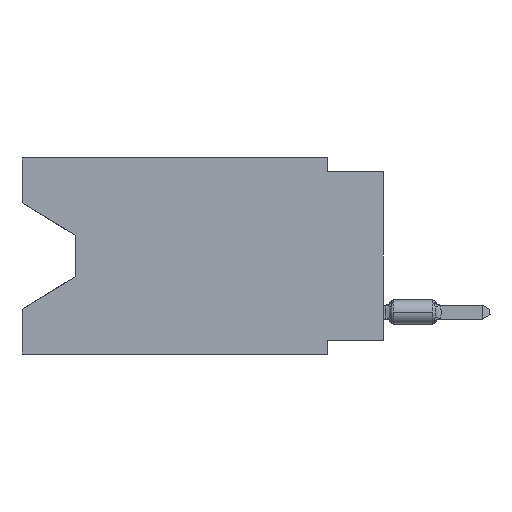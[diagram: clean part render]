
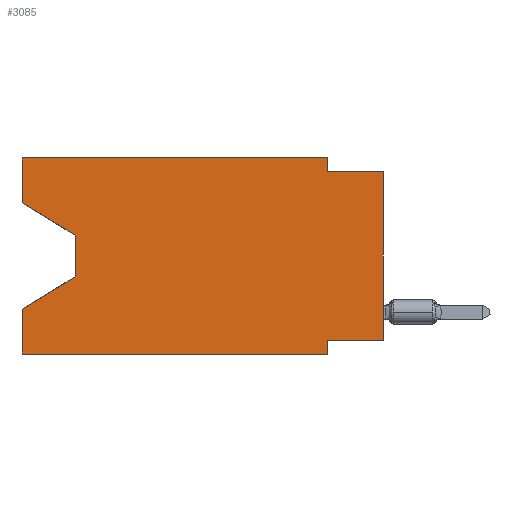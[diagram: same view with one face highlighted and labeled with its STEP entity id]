
A CAD part, left-side view. The second image highlights one B-rep face of the part: STEP entity #3085.
In plain terms, the highlighted planar face has unit normal (-1, 0, 0).
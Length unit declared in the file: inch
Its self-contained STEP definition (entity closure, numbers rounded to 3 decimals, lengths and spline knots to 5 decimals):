
#94 = ORIENTED_EDGE ( 'NONE', *, *, #30604, .T. ) ;
#130 = EDGE_CURVE ( 'NONE', #18713, #2968, #31496, .T. ) ;
#523 = EDGE_CURVE ( 'NONE', #37211, #47899, #14336, .T. ) ;
#1153 = PLANE ( 'NONE',  #53419 ) ;
#2968 = VERTEX_POINT ( 'NONE', #8734 ) ;
#3085 = ADVANCED_FACE ( 'NONE', ( #48333 ), #1153, .F. ) ;
#3210 = EDGE_CURVE ( 'NONE', #29739, #53073, #45524, .T. ) ;
#3439 = ORIENTED_EDGE ( 'NONE', *, *, #51455, .F. ) ;
#4530 = CARTESIAN_POINT ( 'NONE',  ( 0., 0.55, -0.138 ) ) ;
#4760 = VECTOR ( 'NONE', #29917, 39.37008 ) ;
#5023 = VECTOR ( 'NONE', #26754, 39.37008 ) ;
#5620 = CARTESIAN_POINT ( 'NONE',  ( 0., 0.645, 0. ) ) ;
#5748 = VECTOR ( 'NONE', #40285, 39.37008 ) ;
#6847 = CARTESIAN_POINT ( 'NONE',  ( 0., 0.645, -0.35 ) ) ;
#7957 = VECTOR ( 'NONE', #19310, 39.37008 ) ;
#8463 = EDGE_CURVE ( 'NONE', #39669, #2968, #15248, .T. ) ;
#8488 = ORIENTED_EDGE ( 'NONE', *, *, #130, .F. ) ;
#8734 = CARTESIAN_POINT ( 'NONE',  ( 0., 0.1, -0.35 ) ) ;
#9018 = DIRECTION ( 'NONE',  ( 1., 0., 0. ) ) ;
#10487 = VERTEX_POINT ( 'NONE', #49384 ) ;
#11564 = CARTESIAN_POINT ( 'NONE',  ( 0., 0., 0. ) ) ;
#11625 = DIRECTION ( 'NONE',  ( 0., -1., 0. ) ) ;
#11830 = DIRECTION ( 'NONE',  ( 0., 0., 1. ) ) ;
#12319 = EDGE_CURVE ( 'NONE', #44673, #18713, #16923, .T. ) ;
#12604 = CARTESIAN_POINT ( 'NONE',  ( 0., 0.645, -0.26975 ) ) ;
#12616 = VERTEX_POINT ( 'NONE', #41157 ) ;
#12770 = ORIENTED_EDGE ( 'NONE', *, *, #37402, .F. ) ;
#13154 = VECTOR ( 'NONE', #42309, 39.37008 ) ;
#13307 = ORIENTED_EDGE ( 'NONE', *, *, #8463, .T. ) ;
#13615 = DIRECTION ( 'NONE',  ( 0., 0., -1. ) ) ;
#13728 = VECTOR ( 'NONE', #30516, 39.37008 ) ;
#14162 = LINE ( 'NONE', #11564, #27869 ) ;
#14187 = CARTESIAN_POINT ( 'NONE',  ( 0., 0.1, -0.35 ) ) ;
#14336 = LINE ( 'NONE', #40005, #36275 ) ;
#14960 = VERTEX_POINT ( 'NONE', #54666 ) ;
#15107 = CARTESIAN_POINT ( 'NONE',  ( 0., 0.645, 0. ) ) ;
#15248 = LINE ( 'NONE', #6847, #40459 ) ;
#15988 = CARTESIAN_POINT ( 'NONE',  ( 0., 0.645, 0. ) ) ;
#16197 = LINE ( 'NONE', #15107, #30151 ) ;
#16202 = EDGE_CURVE ( 'NONE', #12616, #10487, #16197, .T. ) ;
#16923 = LINE ( 'NONE', #30054, #13154 ) ;
#17351 = CARTESIAN_POINT ( 'NONE',  ( 0., 0.645, 0. ) ) ;
#18445 = ORIENTED_EDGE ( 'NONE', *, *, #3210, .T. ) ;
#18713 = VERTEX_POINT ( 'NONE', #23913 ) ;
#18798 = LINE ( 'NONE', #20107, #5748 ) ;
#19310 = DIRECTION ( 'NONE',  ( 0., 0.855, -0.519 ) ) ;
#20107 = CARTESIAN_POINT ( 'NONE',  ( 0., 0.645, -0.08025 ) ) ;
#20171 = CARTESIAN_POINT ( 'NONE',  ( 0., 0.1, -0.025 ) ) ;
#22946 = CARTESIAN_POINT ( 'NONE',  ( 0., 0.55, -0.212 ) ) ;
#23913 = CARTESIAN_POINT ( 'NONE',  ( 0., 0.1, -0.325 ) ) ;
#25300 = CARTESIAN_POINT ( 'NONE',  ( 0., 0.55, -0.138 ) ) ;
#25335 = LINE ( 'NONE', #51583, #49440 ) ;
#25859 = ORIENTED_EDGE ( 'NONE', *, *, #26930, .F. ) ;
#26754 = DIRECTION ( 'NONE',  ( 0., 0., -1. ) ) ;
#26930 = EDGE_CURVE ( 'NONE', #10487, #37211, #25335, .T. ) ;
#27163 = DIRECTION ( 'NONE',  ( 0., -1., 0. ) ) ;
#27730 = EDGE_LOOP ( 'NONE', ( #47779, #94, #18445, #3439, #13307, #8488, #44614, #50580, #31927, #25859, #44111, #12770 ) ) ;
#27869 = VECTOR ( 'NONE', #11830, 39.37008 ) ;
#29739 = VERTEX_POINT ( 'NONE', #46267 ) ;
#29917 = DIRECTION ( 'NONE',  ( 0., 0., 1. ) ) ;
#30054 = CARTESIAN_POINT ( 'NONE',  ( 0., 0., -0.325 ) ) ;
#30151 = VECTOR ( 'NONE', #40781, 39.37008 ) ;
#30516 = DIRECTION ( 'NONE',  ( 0., 0., -1. ) ) ;
#30604 = EDGE_CURVE ( 'NONE', #35213, #29739, #34432, .T. ) ;
#31496 = LINE ( 'NONE', #14187, #5023 ) ;
#31927 = ORIENTED_EDGE ( 'NONE', *, *, #523, .F. ) ;
#34432 = LINE ( 'NONE', #4530, #13728 ) ;
#35213 = VERTEX_POINT ( 'NONE', #25300 ) ;
#36275 = VECTOR ( 'NONE', #27163, 39.37008 ) ;
#37211 = VERTEX_POINT ( 'NONE', #20171 ) ;
#37402 = EDGE_CURVE ( 'NONE', #14960, #12616, #38022, .T. ) ;
#37890 = CARTESIAN_POINT ( 'NONE',  ( 0., 0.645, -0.35 ) ) ;
#38022 = LINE ( 'NONE', #17351, #4760 ) ;
#38048 = DIRECTION ( 'NONE',  ( 0., 0., 1. ) ) ;
#39031 = EDGE_CURVE ( 'NONE', #14960, #35213, #18798, .T. ) ;
#39360 = VECTOR ( 'NONE', #38048, 39.37008 ) ;
#39669 = VERTEX_POINT ( 'NONE', #37890 ) ;
#40005 = CARTESIAN_POINT ( 'NONE',  ( 0., 0., -0.025 ) ) ;
#40285 = DIRECTION ( 'NONE',  ( 0., -0.855, -0.519 ) ) ;
#40459 = VECTOR ( 'NONE', #11625, 39.37008 ) ;
#40781 = DIRECTION ( 'NONE',  ( 0., -1., 0. ) ) ;
#41157 = CARTESIAN_POINT ( 'NONE',  ( 0., 0.645, 0. ) ) ;
#41734 = CARTESIAN_POINT ( 'NONE',  ( 0., 0., -0.025 ) ) ;
#42309 = DIRECTION ( 'NONE',  ( 0., 1., 0. ) ) ;
#43603 = DIRECTION ( 'NONE',  ( 0., 0., -1. ) ) ;
#44111 = ORIENTED_EDGE ( 'NONE', *, *, #16202, .F. ) ;
#44614 = ORIENTED_EDGE ( 'NONE', *, *, #12319, .F. ) ;
#44673 = VERTEX_POINT ( 'NONE', #46372 ) ;
#45524 = LINE ( 'NONE', #22946, #7957 ) ;
#46267 = CARTESIAN_POINT ( 'NONE',  ( 0., 0.55, -0.212 ) ) ;
#46372 = CARTESIAN_POINT ( 'NONE',  ( 0., 0., -0.325 ) ) ;
#46963 = LINE ( 'NONE', #15988, #39360 ) ;
#47779 = ORIENTED_EDGE ( 'NONE', *, *, #39031, .T. ) ;
#47899 = VERTEX_POINT ( 'NONE', #41734 ) ;
#48333 = FACE_OUTER_BOUND ( 'NONE', #27730, .T. ) ;
#49384 = CARTESIAN_POINT ( 'NONE',  ( 0., 0.1, 0. ) ) ;
#49440 = VECTOR ( 'NONE', #13615, 39.37008 ) ;
#50580 = ORIENTED_EDGE ( 'NONE', *, *, #52614, .T. ) ;
#51455 = EDGE_CURVE ( 'NONE', #39669, #53073, #46963, .T. ) ;
#51583 = CARTESIAN_POINT ( 'NONE',  ( 0., 0.1, 0. ) ) ;
#52614 = EDGE_CURVE ( 'NONE', #44673, #47899, #14162, .T. ) ;
#53073 = VERTEX_POINT ( 'NONE', #12604 ) ;
#53419 = AXIS2_PLACEMENT_3D ( 'NONE', #5620, #9018, #43603 ) ;
#54666 = CARTESIAN_POINT ( 'NONE',  ( 0., 0.645, -0.08025 ) ) ;
